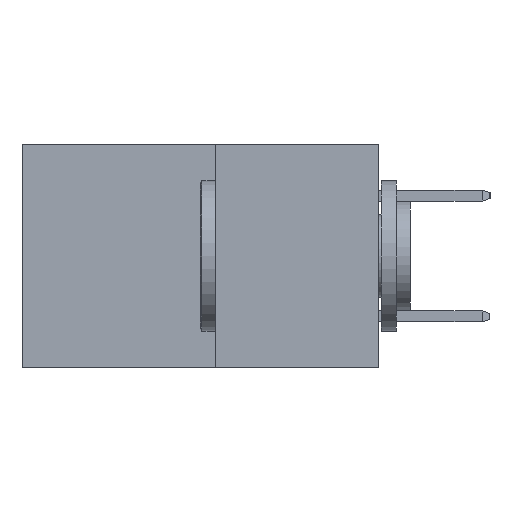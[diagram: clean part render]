
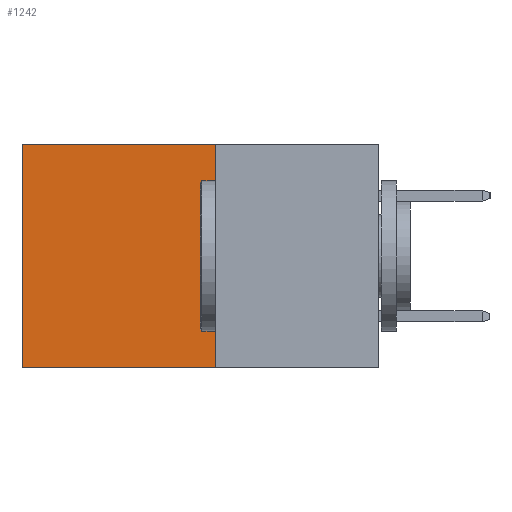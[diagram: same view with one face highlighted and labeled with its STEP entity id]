
A CAD part, left-side view. The second image highlights one B-rep face of the part: STEP entity #1242.
In plain terms, the highlighted planar face has unit normal (-1, 0, 0).
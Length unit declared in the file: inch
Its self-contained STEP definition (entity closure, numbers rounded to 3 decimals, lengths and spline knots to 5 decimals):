
#604 = LINE ( 'NONE', #8521, #8776 ) ;
#872 = CARTESIAN_POINT ( 'NONE',  ( 0.277, 0.59, 0. ) ) ;
#1242 = ADVANCED_FACE ( 'NONE', ( #4103 ), #5076, .F. ) ;
#1599 = ORIENTED_EDGE ( 'NONE', *, *, #9689, .T. ) ;
#1612 = CARTESIAN_POINT ( 'NONE',  ( 0.277, 0.27, -0.37 ) ) ;
#1742 = CARTESIAN_POINT ( 'NONE',  ( 0.277, 0.27, -0.37 ) ) ;
#1864 = VERTEX_POINT ( 'NONE', #2984 ) ;
#2672 = EDGE_CURVE ( 'NONE', #9594, #9561, #7028, .T. ) ;
#2984 = CARTESIAN_POINT ( 'NONE',  ( 0.277, 0.27, 0. ) ) ;
#3391 = CARTESIAN_POINT ( 'NONE',  ( 0.277, 0.59, -0.37 ) ) ;
#3548 = VERTEX_POINT ( 'NONE', #872 ) ;
#4103 = FACE_OUTER_BOUND ( 'NONE', #8869, .T. ) ;
#4732 = EDGE_CURVE ( 'NONE', #1864, #3548, #604, .T. ) ;
#5047 = DIRECTION ( 'NONE',  ( 1., 0., 0. ) ) ;
#5076 = PLANE ( 'NONE',  #6644 ) ;
#5884 = ORIENTED_EDGE ( 'NONE', *, *, #2672, .F. ) ;
#6116 = DIRECTION ( 'NONE',  ( 0., 1., 0. ) ) ;
#6120 = ORIENTED_EDGE ( 'NONE', *, *, #4732, .T. ) ;
#6295 = VECTOR ( 'NONE', #6116, 39.37008 ) ;
#6601 = DIRECTION ( 'NONE',  ( 0., 0., -1. ) ) ;
#6644 = AXIS2_PLACEMENT_3D ( 'NONE', #9060, #5047, #6601 ) ;
#6817 = VECTOR ( 'NONE', #7862, 39.37008 ) ;
#7028 = LINE ( 'NONE', #1742, #6295 ) ;
#7102 = VECTOR ( 'NONE', #8076, 39.37008 ) ;
#7611 = EDGE_CURVE ( 'NONE', #1864, #9594, #8833, .T. ) ;
#7862 = DIRECTION ( 'NONE',  ( 0., 0., -1. ) ) ;
#7908 = ORIENTED_EDGE ( 'NONE', *, *, #7611, .F. ) ;
#7974 = CARTESIAN_POINT ( 'NONE',  ( 0.277, 0.27, -0.37 ) ) ;
#8076 = DIRECTION ( 'NONE',  ( 0., 0., -1. ) ) ;
#8521 = CARTESIAN_POINT ( 'NONE',  ( 0.277, 0.27, 0. ) ) ;
#8546 = DIRECTION ( 'NONE',  ( 0., 1., 0. ) ) ;
#8776 = VECTOR ( 'NONE', #8546, 39.37008 ) ;
#8833 = LINE ( 'NONE', #7974, #6817 ) ;
#8869 = EDGE_LOOP ( 'NONE', ( #1599, #5884, #7908, #6120 ) ) ;
#9060 = CARTESIAN_POINT ( 'NONE',  ( 0.277, 0.27, -0.37 ) ) ;
#9105 = LINE ( 'NONE', #3391, #7102 ) ;
#9561 = VERTEX_POINT ( 'NONE', #10120 ) ;
#9594 = VERTEX_POINT ( 'NONE', #1612 ) ;
#9689 = EDGE_CURVE ( 'NONE', #3548, #9561, #9105, .T. ) ;
#10120 = CARTESIAN_POINT ( 'NONE',  ( 0.277, 0.59, -0.37 ) ) ;
